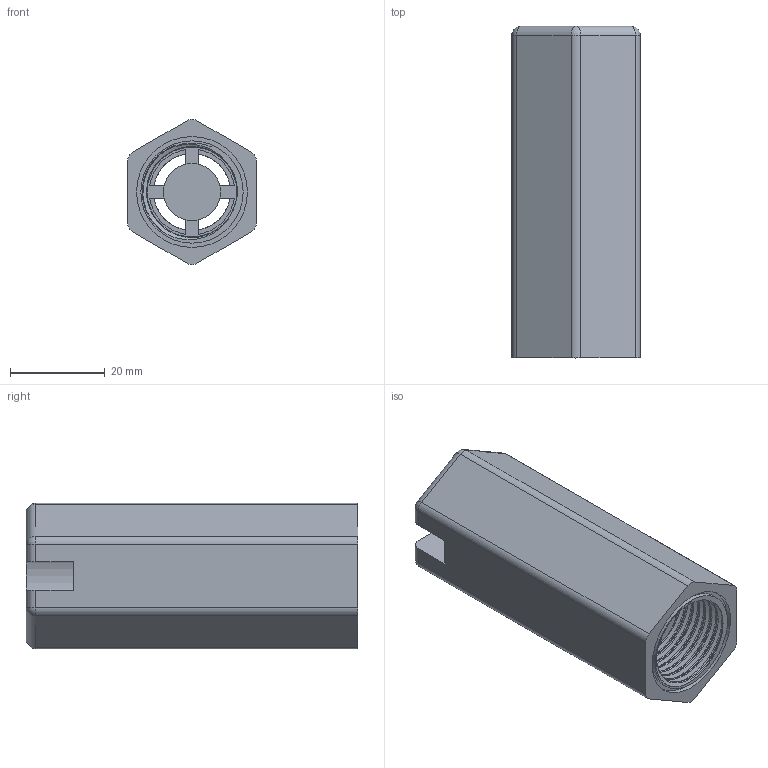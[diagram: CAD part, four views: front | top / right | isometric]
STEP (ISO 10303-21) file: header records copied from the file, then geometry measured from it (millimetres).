
FILE_DESCRIPTION(/* description */ (''),/* implementation_level */ '2;1');
FILE_NAME(/* name */ 'Fitting for 6mm Rod - Loose Fit.stp',/* time_stamp */ '2019-12-08T14:45:50-06:00',/* author */ ('johne'),/* organization */ (''),/* preprocessor_version */ 'ST-DEVELOPER v18',/* originating_system */ 'Autodesk Inventor 2020',/* authorisation */ '');
FILE_SCHEMA (('AUTOMOTIVE_DESIGN { 1 0 10303 214 3 1 1 }'));
Length unit declared in the file: millimetre
Products named in the file (1): Fitting for 6mm Rod
Bounding box: 27.05 x 69.85 x 30.61 mm (x, y, z)
Volume: 28354.9 mm3; surface area: 14369.1 mm2
Topology: 1 solids, 1 shells, 110 faces, 322 edges, 213 vertices
Faces by surface type: cylinder 51, plane 41, torus 6, sphere 6, bspline 6
Full cylindrical faces by diameter (mm): 6.005 x1, 12 x1, 16.2 x2, 20.955 x13, 21.546 x1, 23.344 x1
Entity records: 10813 total; most frequent: CARTESIAN_POINT 7936, ORIENTED_EDGE 644, DIRECTION 534, EDGE_CURVE 322, VERTEX_POINT 213, AXIS2_PLACEMENT_3D 200, LINE 134, VECTOR 134
